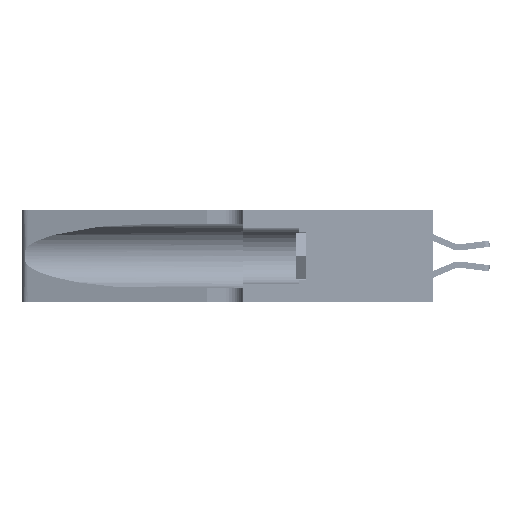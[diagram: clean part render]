
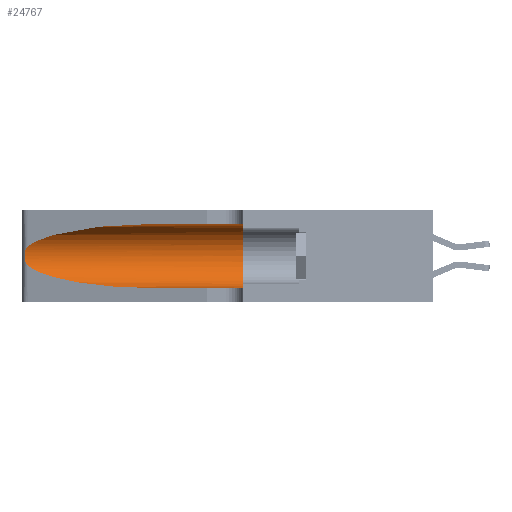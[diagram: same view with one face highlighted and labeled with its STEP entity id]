
A CAD part, left-side view. The second image highlights one B-rep face of the part: STEP entity #24767.
In plain terms, the highlighted cylindrical face has radius 3.308 mm (diameter 6.617 mm), a partial arc.
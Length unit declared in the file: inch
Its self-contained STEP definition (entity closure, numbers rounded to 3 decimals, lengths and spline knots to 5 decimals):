
#620 =( BOUNDED_CURVE ( )  B_SPLINE_CURVE ( 3, ( #38796, #13982, #4777, #26577 ),
 .UNSPECIFIED., .F., .T. ) 
 B_SPLINE_CURVE_WITH_KNOTS ( ( 4, 4 ),
 ( 1.5708, 2.84003 ),
 .UNSPECIFIED. ) 
 CURVE ( )  GEOMETRIC_REPRESENTATION_ITEM ( )  RATIONAL_B_SPLINE_CURVE ( ( 1., 0.87, 0.87, 1. ) ) 
 REPRESENTATION_ITEM ( '' )  );
#1310 = CARTESIAN_POINT ( 'NONE',  ( 0.26075, 1.23896, 0.19203 ) ) ;
#1372 = CARTESIAN_POINT ( 'NONE',  ( 0.1305, 0.72297, 0.05475 ) ) ;
#1868 = CARTESIAN_POINT ( 'NONE',  ( 0.1305, 1.61858, 0.05475 ) ) ;
#2324 = EDGE_CURVE ( 'NONE', #8041, #31357, #21029, .T. ) ;
#3407 = CARTESIAN_POINT ( 'NONE',  ( 0.1305, 1.61858, 0.31525 ) ) ;
#3498 = ORIENTED_EDGE ( 'NONE', *, *, #19276, .T. ) ;
#4394 = CARTESIAN_POINT ( 'NONE',  ( 0.26017, 1.23833, 0.17102 ) ) ;
#4777 = CARTESIAN_POINT ( 'NONE',  ( 0.2373, 1.15595, 0.28018 ) ) ;
#5533 = VERTEX_POINT ( 'NONE', #30210 ) ;
#7525 = CARTESIAN_POINT ( 'NONE',  ( 0.25789, 1.23486, 0.15765 ) ) ;
#8041 = VERTEX_POINT ( 'NONE', #10106 ) ;
#8139 = LINE ( 'NONE', #1868, #29731 ) ;
#9614 = DIRECTION ( 'NONE',  ( 0., -1., 0. ) ) ;
#10106 = CARTESIAN_POINT ( 'NONE',  ( 0.25487, 1.22718, 0.22369 ) ) ;
#10237 = DIRECTION ( 'NONE',  ( 0., 1., 0. ) ) ;
#10441 = DIRECTION ( 'NONE',  ( 0., 0., -1. ) ) ;
#10541 = CARTESIAN_POINT ( 'NONE',  ( 0.25487, 1.22718, 0.14631 ) ) ;
#10607 = CARTESIAN_POINT ( 'NONE',  ( 0.25555, 1.22993, 0.14849 ) ) ;
#11011 = AXIS2_PLACEMENT_3D ( 'NONE', #28923, #10237, #32006 ) ;
#11716 = VERTEX_POINT ( 'NONE', #20335 ) ;
#13597 = CARTESIAN_POINT ( 'NONE',  ( 0.25487, 1.22718, 0.22369 ) ) ;
#13982 = CARTESIAN_POINT ( 'NONE',  ( 0.18966, 0.96281, 0.31525 ) ) ;
#14309 = DIRECTION ( 'NONE',  ( 0., -1., 0. ) ) ;
#14575 = ORIENTED_EDGE ( 'NONE', *, *, #2324, .T. ) ;
#16756 = CARTESIAN_POINT ( 'NONE',  ( 0.25787, 1.23484, 0.2124 ) ) ;
#16836 = DIRECTION ( 'NONE',  ( 0., -1., 0. ) ) ;
#17276 = CYLINDRICAL_SURFACE ( 'NONE', #27672, 0.13025 ) ;
#18287 = FACE_OUTER_BOUND ( 'NONE', #34729, .T. ) ;
#19276 = EDGE_CURVE ( 'NONE', #31357, #5533, #36662, .T. ) ;
#19810 = VERTEX_POINT ( 'NONE', #28507 ) ;
#19880 = CARTESIAN_POINT ( 'NONE',  ( 0.1305, 0.72297, 0.31525 ) ) ;
#19895 = CARTESIAN_POINT ( 'NONE',  ( 0.26018, 1.23835, 0.19895 ) ) ;
#19954 = CARTESIAN_POINT ( 'NONE',  ( 0.18966, 0.96281, 0.05475 ) ) ;
#20335 = CARTESIAN_POINT ( 'NONE',  ( 0.1305, 0.35, 0.31525 ) ) ;
#20934 = EDGE_CURVE ( 'NONE', #37078, #11716, #23959, .T. ) ;
#21029 = B_SPLINE_CURVE_WITH_KNOTS ( 'NONE', 3,
 ( #13597, #38279, #32255, #16756, #38418, #19895, #1310, #23061, #4394, #26185, #7525, #29278, #10607, #32390 ),
 .UNSPECIFIED., .F., .F.,
 ( 4, 2, 2, 2, 2, 2, 4 ),
 ( 0., 0.00027, 0.00053, 0.00107, 0.0016, 0.00187, 0.00214 ),
 .UNSPECIFIED. ) ;
#22979 = VECTOR ( 'NONE', #9614, 39.37008 ) ;
#23061 = CARTESIAN_POINT ( 'NONE',  ( 0.26075, 1.23896, 0.178 ) ) ;
#23959 = LINE ( 'NONE', #3407, #22979 ) ;
#24767 = ADVANCED_FACE ( 'NONE', ( #18287 ), #17276, .F. ) ;
#25954 = CIRCLE ( 'NONE', #11011, 0.13025 ) ;
#26185 = CARTESIAN_POINT ( 'NONE',  ( 0.25856, 1.23593, 0.16098 ) ) ;
#26577 = CARTESIAN_POINT ( 'NONE',  ( 0.25487, 1.22718, 0.22369 ) ) ;
#26753 = ORIENTED_EDGE ( 'NONE', *, *, #27479, .T. ) ;
#27328 = ORIENTED_EDGE ( 'NONE', *, *, #38298, .F. ) ;
#27479 = EDGE_CURVE ( 'NONE', #37078, #8041, #620, .T. ) ;
#27672 = AXIS2_PLACEMENT_3D ( 'NONE', #29379, #16836, #10441 ) ;
#28507 = CARTESIAN_POINT ( 'NONE',  ( 0.1305, 0.35, 0.05475 ) ) ;
#28923 = CARTESIAN_POINT ( 'NONE',  ( 0.1305, 0.35, 0.185 ) ) ;
#29278 = CARTESIAN_POINT ( 'NONE',  ( 0.25639, 1.23186, 0.15144 ) ) ;
#29379 = CARTESIAN_POINT ( 'NONE',  ( 0.1305, 1.61858, 0.185 ) ) ;
#29547 = ORIENTED_EDGE ( 'NONE', *, *, #20934, .F. ) ;
#29623 = CARTESIAN_POINT ( 'NONE',  ( 0.25487, 1.22718, 0.14631 ) ) ;
#29731 = VECTOR ( 'NONE', #14309, 39.37008 ) ;
#30210 = CARTESIAN_POINT ( 'NONE',  ( 0.1305, 0.72297, 0.05475 ) ) ;
#31357 = VERTEX_POINT ( 'NONE', #29623 ) ;
#32006 = DIRECTION ( 'NONE',  ( 0., 0., 1. ) ) ;
#32064 = EDGE_CURVE ( 'NONE', #5533, #19810, #8139, .T. ) ;
#32255 = CARTESIAN_POINT ( 'NONE',  ( 0.25639, 1.23184, 0.21858 ) ) ;
#32390 = CARTESIAN_POINT ( 'NONE',  ( 0.25487, 1.22718, 0.14631 ) ) ;
#34729 = EDGE_LOOP ( 'NONE', ( #26753, #14575, #3498, #36671, #27328, #29547 ) ) ;
#35406 = CARTESIAN_POINT ( 'NONE',  ( 0.2373, 1.15595, 0.08982 ) ) ;
#36662 =( BOUNDED_CURVE ( )  B_SPLINE_CURVE ( 3, ( #10541, #35406, #19954, #1372 ),
 .UNSPECIFIED., .F., .F. ) 
 B_SPLINE_CURVE_WITH_KNOTS ( ( 4, 4 ),
 ( 3.44316, 4.71239 ),
 .UNSPECIFIED. ) 
 CURVE ( )  GEOMETRIC_REPRESENTATION_ITEM ( )  RATIONAL_B_SPLINE_CURVE ( ( 1., 0.87, 0.87, 1. ) ) 
 REPRESENTATION_ITEM ( '' )  );
#36671 = ORIENTED_EDGE ( 'NONE', *, *, #32064, .T. ) ;
#37078 = VERTEX_POINT ( 'NONE', #19880 ) ;
#38279 = CARTESIAN_POINT ( 'NONE',  ( 0.25555, 1.22994, 0.2215 ) ) ;
#38298 = EDGE_CURVE ( 'NONE', #11716, #19810, #25954, .T. ) ;
#38418 = CARTESIAN_POINT ( 'NONE',  ( 0.25854, 1.2359, 0.20912 ) ) ;
#38796 = CARTESIAN_POINT ( 'NONE',  ( 0.1305, 0.72297, 0.31525 ) ) ;
